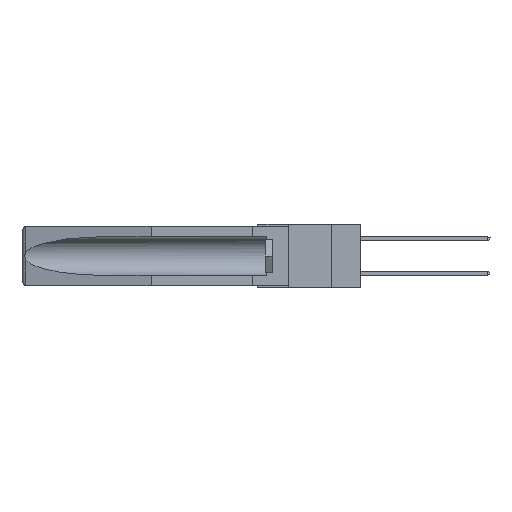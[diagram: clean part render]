
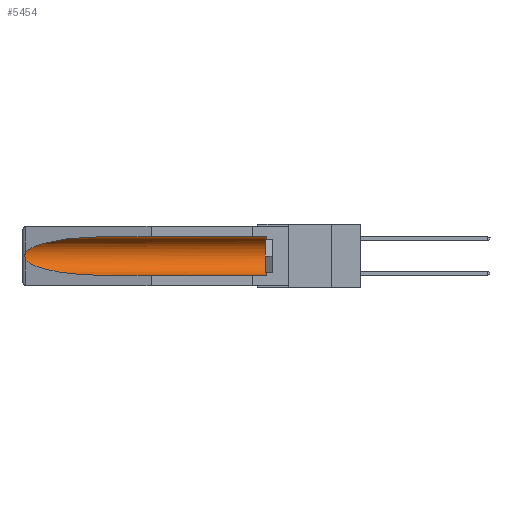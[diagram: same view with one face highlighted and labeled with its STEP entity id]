
A CAD part, left-side view. The second image highlights one B-rep face of the part: STEP entity #5454.
In plain terms, the highlighted cylindrical face has radius 2.857 mm (diameter 5.715 mm), a partial arc.
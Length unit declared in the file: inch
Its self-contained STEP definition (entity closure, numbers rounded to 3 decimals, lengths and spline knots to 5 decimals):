
#45 = ORIENTED_EDGE ( 'NONE', *, *, #5758, .T. ) ;
#304 = EDGE_CURVE ( 'NONE', #7981, #4498, #4572, .T. ) ;
#312 = CARTESIAN_POINT ( 'NONE',  ( 0.155, 0.126, -0.1715 ) ) ;
#622 = FACE_OUTER_BOUND ( 'NONE', #10912, .T. ) ;
#904 = CARTESIAN_POINT ( 'NONE',  ( 0.26537, 1.52718, -0.14972 ) ) ;
#1302 = CARTESIAN_POINT ( 'NONE',  ( 0.155, 1.07973, -0.059 ) ) ;
#1311 =( BOUNDED_CURVE ( )  B_SPLINE_CURVE ( 3, ( #7159, #2345, #5444, #904 ),
 .UNSPECIFIED., .F., .T. ) 
 B_SPLINE_CURVE_WITH_KNOTS ( ( 4, 4 ),
 ( 4.71239, 6.08839 ),
 .UNSPECIFIED. ) 
 CURVE ( )  GEOMETRIC_REPRESENTATION_ITEM ( )  RATIONAL_B_SPLINE_CURVE ( ( 1., 0.848, 0.848, 1. ) ) 
 REPRESENTATION_ITEM ( '' )  );
#1320 = DIRECTION ( 'NONE',  ( 0., 0., 1. ) ) ;
#1887 = DIRECTION ( 'NONE',  ( 0., -1., 0. ) ) ;
#2198 = ORIENTED_EDGE ( 'NONE', *, *, #6536, .T. ) ;
#2345 = CARTESIAN_POINT ( 'NONE',  ( 0.21114, 1.30732, -0.059 ) ) ;
#2434 = ORIENTED_EDGE ( 'NONE', *, *, #2575, .T. ) ;
#2575 = EDGE_CURVE ( 'NONE', #2879, #11392, #4592, .T. ) ;
#2812 = CARTESIAN_POINT ( 'NONE',  ( 0.155, 0.126, -0.284 ) ) ;
#2879 = VERTEX_POINT ( 'NONE', #17720 ) ;
#3450 = DIRECTION ( 'NONE',  ( 0., 0., 1. ) ) ;
#3946 = VERTEX_POINT ( 'NONE', #2812 ) ;
#4063 = CARTESIAN_POINT ( 'NONE',  ( 0.26597, 1.52961, -0.15275 ) ) ;
#4498 = VERTEX_POINT ( 'NONE', #18703 ) ;
#4572 = B_SPLINE_CURVE_WITH_KNOTS ( 'NONE', 3,
 ( #10323, #4063, #15098, #15035, #8823, #19759, #6967, #19492, #8622, #11713 ),
 .UNSPECIFIED., .F., .F.,
 ( 4, 2, 2, 2, 4 ),
 ( 0., 0.00029, 0.00058, 0.00087, 0.00117 ),
 .UNSPECIFIED. ) ;
#4592 = LINE ( 'NONE', #6683, #12693 ) ;
#5032 = VERTEX_POINT ( 'NONE', #19584 ) ;
#5444 = CARTESIAN_POINT ( 'NONE',  ( 0.25451, 1.48313, -0.09465 ) ) ;
#5454 = ADVANCED_FACE ( 'NONE', ( #622 ), #20245, .F. ) ;
#5758 = EDGE_CURVE ( 'NONE', #3946, #2879, #7747, .T. ) ;
#6536 = EDGE_CURVE ( 'NONE', #11392, #7981, #1311, .T. ) ;
#6683 = CARTESIAN_POINT ( 'NONE',  ( 0.155, -0.30754, -0.059 ) ) ;
#6967 = CARTESIAN_POINT ( 'NONE',  ( 0.2673, 1.53269, -0.17917 ) ) ;
#7159 = CARTESIAN_POINT ( 'NONE',  ( 0.155, 1.07973, -0.059 ) ) ;
#7365 = CARTESIAN_POINT ( 'NONE',  ( 0.155, 1.07973, -0.284 ) ) ;
#7428 = CARTESIAN_POINT ( 'NONE',  ( 0.21114, 1.30732, -0.284 ) ) ;
#7747 = CIRCLE ( 'NONE', #13500, 0.1125 ) ;
#7981 = VERTEX_POINT ( 'NONE', #10501 ) ;
#8622 = CARTESIAN_POINT ( 'NONE',  ( 0.26597, 1.5296, -0.19026 ) ) ;
#8823 = CARTESIAN_POINT ( 'NONE',  ( 0.2675, 1.53308, -0.16763 ) ) ;
#9459 = ORIENTED_EDGE ( 'NONE', *, *, #304, .T. ) ;
#10035 = CARTESIAN_POINT ( 'NONE',  ( 0.26537, 1.52718, -0.19328 ) ) ;
#10115 =( BOUNDED_CURVE ( )  B_SPLINE_CURVE ( 3, ( #10035, #17825, #7428, #7365 ),
 .UNSPECIFIED., .F., .F. ) 
 B_SPLINE_CURVE_WITH_KNOTS ( ( 4, 4 ),
 ( 0.1948, 1.5708 ),
 .UNSPECIFIED. ) 
 CURVE ( )  GEOMETRIC_REPRESENTATION_ITEM ( )  RATIONAL_B_SPLINE_CURVE ( ( 1., 0.848, 0.848, 1. ) ) 
 REPRESENTATION_ITEM ( '' )  );
#10323 = CARTESIAN_POINT ( 'NONE',  ( 0.26537, 1.52718, -0.14972 ) ) ;
#10501 = CARTESIAN_POINT ( 'NONE',  ( 0.26537, 1.52718, -0.14972 ) ) ;
#10721 = ORIENTED_EDGE ( 'NONE', *, *, #12204, .F. ) ;
#10912 = EDGE_LOOP ( 'NONE', ( #2198, #9459, #12594, #10721, #45, #2434 ) ) ;
#11392 = VERTEX_POINT ( 'NONE', #1302 ) ;
#11713 = CARTESIAN_POINT ( 'NONE',  ( 0.26537, 1.52718, -0.19328 ) ) ;
#12099 = CARTESIAN_POINT ( 'NONE',  ( 0.155, -0.30754, -0.1715 ) ) ;
#12204 = EDGE_CURVE ( 'NONE', #3946, #5032, #16284, .T. ) ;
#12594 = ORIENTED_EDGE ( 'NONE', *, *, #17146, .T. ) ;
#12693 = VECTOR ( 'NONE', #15022, 39.37008 ) ;
#13500 = AXIS2_PLACEMENT_3D ( 'NONE', #312, #1887, #3450 ) ;
#15022 = DIRECTION ( 'NONE',  ( 0., 1., 0. ) ) ;
#15035 = CARTESIAN_POINT ( 'NONE',  ( 0.2673, 1.5327, -0.16383 ) ) ;
#15098 = CARTESIAN_POINT ( 'NONE',  ( 0.26654, 1.53092, -0.15636 ) ) ;
#15556 = VECTOR ( 'NONE', #16666, 39.37008 ) ;
#16242 = AXIS2_PLACEMENT_3D ( 'NONE', #12099, #20141, #1320 ) ;
#16284 = LINE ( 'NONE', #16603, #15556 ) ;
#16603 = CARTESIAN_POINT ( 'NONE',  ( 0.155, -0.30754, -0.284 ) ) ;
#16666 = DIRECTION ( 'NONE',  ( 0., 1., 0. ) ) ;
#17146 = EDGE_CURVE ( 'NONE', #4498, #5032, #10115, .T. ) ;
#17720 = CARTESIAN_POINT ( 'NONE',  ( 0.155, 0.126, -0.059 ) ) ;
#17825 = CARTESIAN_POINT ( 'NONE',  ( 0.25451, 1.48313, -0.24835 ) ) ;
#18703 = CARTESIAN_POINT ( 'NONE',  ( 0.26537, 1.52718, -0.19328 ) ) ;
#19492 = CARTESIAN_POINT ( 'NONE',  ( 0.26655, 1.53094, -0.18657 ) ) ;
#19584 = CARTESIAN_POINT ( 'NONE',  ( 0.155, 1.07973, -0.284 ) ) ;
#19759 = CARTESIAN_POINT ( 'NONE',  ( 0.2675, 1.53308, -0.17534 ) ) ;
#20141 = DIRECTION ( 'NONE',  ( 0., 1., 0. ) ) ;
#20245 = CYLINDRICAL_SURFACE ( 'NONE', #16242, 0.1125 ) ;
